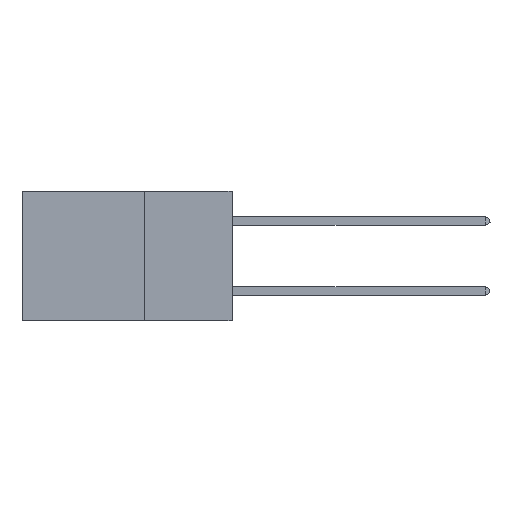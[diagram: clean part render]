
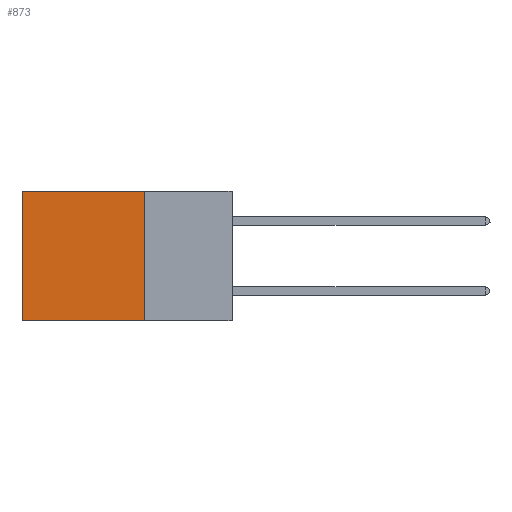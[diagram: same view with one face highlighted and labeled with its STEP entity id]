
A CAD part, left-side view. The second image highlights one B-rep face of the part: STEP entity #873.
In plain terms, the highlighted planar face has unit normal (-1, 0, 0).
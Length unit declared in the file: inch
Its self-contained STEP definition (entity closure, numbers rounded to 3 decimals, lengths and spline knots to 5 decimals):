
#873 = ADVANCED_FACE ( 'NONE', ( #3336 ), #14568, .F. ) ;
#1381 = DIRECTION ( 'NONE',  ( 0., 1., 0. ) ) ;
#1511 = VERTEX_POINT ( 'NONE', #1825 ) ;
#1825 = CARTESIAN_POINT ( 'NONE',  ( 0.2875, 0.25, -0.37 ) ) ;
#2286 = ORIENTED_EDGE ( 'NONE', *, *, #16643, .F. ) ;
#3336 = FACE_OUTER_BOUND ( 'NONE', #21385, .T. ) ;
#4409 = VECTOR ( 'NONE', #1381, 39.37008 ) ;
#4671 = VECTOR ( 'NONE', #5360, 39.37008 ) ;
#5360 = DIRECTION ( 'NONE',  ( 0., 0., -1. ) ) ;
#6354 = LINE ( 'NONE', #10933, #16424 ) ;
#6480 = VERTEX_POINT ( 'NONE', #23405 ) ;
#7442 = VECTOR ( 'NONE', #11589, 39.37008 ) ;
#8425 = CARTESIAN_POINT ( 'NONE',  ( 0.2875, 0.6, -0.37 ) ) ;
#9480 = LINE ( 'NONE', #23846, #4409 ) ;
#9657 = CARTESIAN_POINT ( 'NONE',  ( 0.2875, 0.25, -0.37 ) ) ;
#9842 = VERTEX_POINT ( 'NONE', #11689 ) ;
#10549 = AXIS2_PLACEMENT_3D ( 'NONE', #13941, #13919, #13858 ) ;
#10933 = CARTESIAN_POINT ( 'NONE',  ( 0.2875, 0.6, 0. ) ) ;
#11589 = DIRECTION ( 'NONE',  ( 0., 1., 0. ) ) ;
#11689 = CARTESIAN_POINT ( 'NONE',  ( 0.2875, 0.25, 0. ) ) ;
#12930 = CARTESIAN_POINT ( 'NONE',  ( 0.2875, 0.25, 0. ) ) ;
#13089 = LINE ( 'NONE', #9657, #7442 ) ;
#13858 = DIRECTION ( 'NONE',  ( 0., 0., -1. ) ) ;
#13919 = DIRECTION ( 'NONE',  ( 1., 0., 0. ) ) ;
#13941 = CARTESIAN_POINT ( 'NONE',  ( 0.2875, 0.25, 0. ) ) ;
#14568 = PLANE ( 'NONE',  #10549 ) ;
#15203 = ORIENTED_EDGE ( 'NONE', *, *, #20117, .T. ) ;
#15881 = ORIENTED_EDGE ( 'NONE', *, *, #17859, .F. ) ;
#16332 = VERTEX_POINT ( 'NONE', #8425 ) ;
#16424 = VECTOR ( 'NONE', #23815, 39.37008 ) ;
#16643 = EDGE_CURVE ( 'NONE', #1511, #16332, #13089, .T. ) ;
#17859 = EDGE_CURVE ( 'NONE', #9842, #1511, #19125, .T. ) ;
#19125 = LINE ( 'NONE', #12930, #4671 ) ;
#20117 = EDGE_CURVE ( 'NONE', #6480, #16332, #6354, .T. ) ;
#21268 = ORIENTED_EDGE ( 'NONE', *, *, #24005, .T. ) ;
#21385 = EDGE_LOOP ( 'NONE', ( #15203, #2286, #15881, #21268 ) ) ;
#23405 = CARTESIAN_POINT ( 'NONE',  ( 0.2875, 0.6, 0. ) ) ;
#23815 = DIRECTION ( 'NONE',  ( 0., 0., -1. ) ) ;
#23846 = CARTESIAN_POINT ( 'NONE',  ( 0.2875, 0.25, 0. ) ) ;
#24005 = EDGE_CURVE ( 'NONE', #9842, #6480, #9480, .T. ) ;
